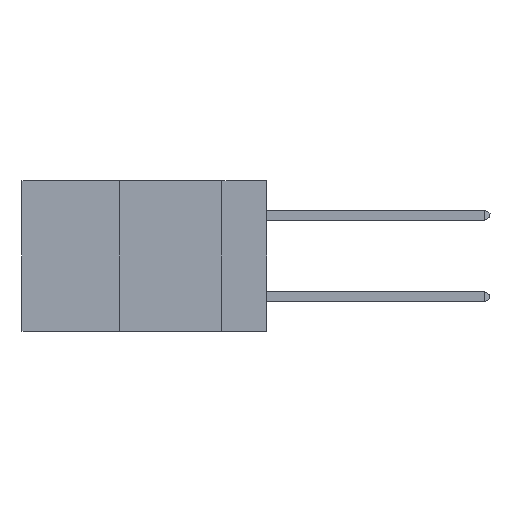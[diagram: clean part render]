
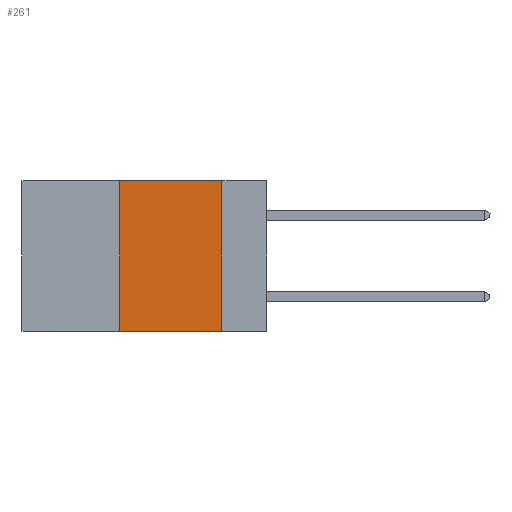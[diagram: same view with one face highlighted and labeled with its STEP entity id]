
A CAD part, left-side view. The second image highlights one B-rep face of the part: STEP entity #261.
In plain terms, the highlighted planar face has unit normal (-1, 0, 0).
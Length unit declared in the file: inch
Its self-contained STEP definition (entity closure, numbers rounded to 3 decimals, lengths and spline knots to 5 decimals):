
#48 = VECTOR ( 'NONE', #2693, 39.37008 ) ;
#261 = ADVANCED_FACE ( 'NONE', ( #4664 ), #2336, .F. ) ;
#406 = VECTOR ( 'NONE', #7689, 39.37008 ) ;
#871 = DIRECTION ( 'NONE',  ( 0., -1., 0. ) ) ;
#1289 = ORIENTED_EDGE ( 'NONE', *, *, #2229, .F. ) ;
#1306 = ORIENTED_EDGE ( 'NONE', *, *, #2954, .F. ) ;
#1499 = CARTESIAN_POINT ( 'NONE',  ( 0., 0.6, 0. ) ) ;
#1553 = CARTESIAN_POINT ( 'NONE',  ( 0., 0.11, 0. ) ) ;
#1814 = CARTESIAN_POINT ( 'NONE',  ( 0., 0.11, -0.37 ) ) ;
#1900 = ORIENTED_EDGE ( 'NONE', *, *, #6036, .F. ) ;
#1943 = ORIENTED_EDGE ( 'NONE', *, *, #4197, .T. ) ;
#2071 = VERTEX_POINT ( 'NONE', #1814 ) ;
#2211 = EDGE_LOOP ( 'NONE', ( #1289, #1306, #1900, #1943 ) ) ;
#2229 = EDGE_CURVE ( 'NONE', #5478, #2071, #4154, .T. ) ;
#2244 = DIRECTION ( 'NONE',  ( 0., 0., -1. ) ) ;
#2312 = CARTESIAN_POINT ( 'NONE',  ( 0., 0.36, -0.37 ) ) ;
#2336 = PLANE ( 'NONE',  #3233 ) ;
#2636 = LINE ( 'NONE', #5227, #4187 ) ;
#2680 = LINE ( 'NONE', #9512, #406 ) ;
#2693 = DIRECTION ( 'NONE',  ( 0., 0., -1. ) ) ;
#2697 = CARTESIAN_POINT ( 'NONE',  ( 0., 0.6, 0. ) ) ;
#2954 = EDGE_CURVE ( 'NONE', #7482, #5478, #7186, .T. ) ;
#3233 = AXIS2_PLACEMENT_3D ( 'NONE', #2697, #5230, #2244 ) ;
#4154 = LINE ( 'NONE', #1553, #48 ) ;
#4187 = VECTOR ( 'NONE', #7333, 39.37008 ) ;
#4197 = EDGE_CURVE ( 'NONE', #4617, #2071, #2680, .T. ) ;
#4617 = VERTEX_POINT ( 'NONE', #2312 ) ;
#4664 = FACE_OUTER_BOUND ( 'NONE', #2211, .T. ) ;
#5227 = CARTESIAN_POINT ( 'NONE',  ( 0., 0.36, 0. ) ) ;
#5230 = DIRECTION ( 'NONE',  ( 1., 0., 0. ) ) ;
#5235 = CARTESIAN_POINT ( 'NONE',  ( 0., 0.11, 0. ) ) ;
#5478 = VERTEX_POINT ( 'NONE', #5235 ) ;
#6034 = CARTESIAN_POINT ( 'NONE',  ( 0., 0.36, 0. ) ) ;
#6036 = EDGE_CURVE ( 'NONE', #4617, #7482, #2636, .T. ) ;
#7186 = LINE ( 'NONE', #1499, #8825 ) ;
#7333 = DIRECTION ( 'NONE',  ( 0., 0., 1. ) ) ;
#7482 = VERTEX_POINT ( 'NONE', #6034 ) ;
#7689 = DIRECTION ( 'NONE',  ( 0., -1., 0. ) ) ;
#8825 = VECTOR ( 'NONE', #871, 39.37008 ) ;
#9512 = CARTESIAN_POINT ( 'NONE',  ( 0., 0.6, -0.37 ) ) ;
